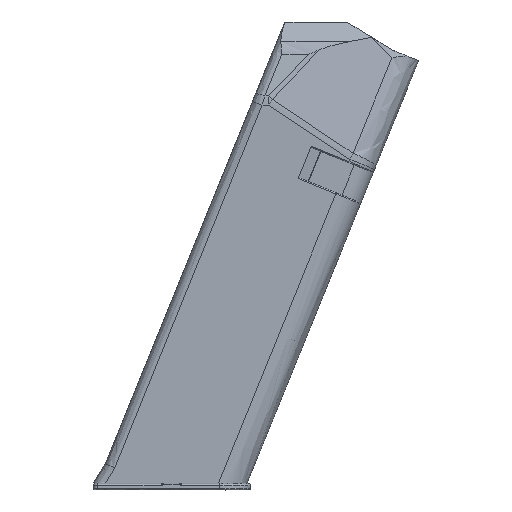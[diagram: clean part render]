
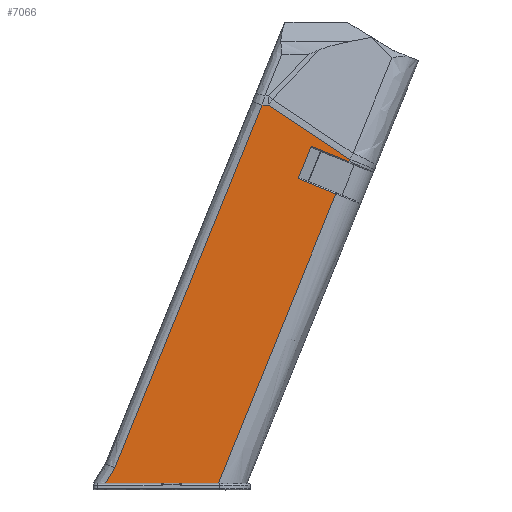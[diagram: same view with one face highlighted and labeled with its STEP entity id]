
A CAD part, top view. The second image highlights one B-rep face of the part: STEP entity #7066.
In plain terms, the highlighted planar face has unit normal (0, 0, 1).
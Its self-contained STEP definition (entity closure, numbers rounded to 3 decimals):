
#513=PLANE('',#7596);
#557=LINE('',#9516,#1223);
#1143=LINE('',#13379,#1809);
#1144=LINE('',#13438,#1810);
#1145=LINE('',#13441,#1811);
#1146=LINE('',#13443,#1812);
#1147=LINE('',#13445,#1813);
#1148=LINE('',#13447,#1814);
#1149=LINE('',#13449,#1815);
#1150=LINE('',#13451,#1816);
#1151=LINE('',#13452,#1817);
#1223=VECTOR('',#7720,982.236);
#1809=VECTOR('',#9110,10.);
#1810=VECTOR('',#9111,10.);
#1811=VECTOR('',#9114,1030.);
#1812=VECTOR('',#9115,975.);
#1813=VECTOR('',#9116,1030.);
#1814=VECTOR('',#9117,977.064);
#1815=VECTOR('',#9118,982.236);
#1816=VECTOR('',#9119,1030.);
#1817=VECTOR('',#9120,1028.422);
#2219=FACE_OUTER_BOUND('',#2621,.T.);
#2621=EDGE_LOOP('',(#6284,#6285,#6286,#6287,#6288,#6289,#6290,#6291,#6292,
#6293));
#2916=VERTEX_POINT('',#9513);
#2917=VERTEX_POINT('',#9515);
#3502=VERTEX_POINT('',#13372);
#3505=VERTEX_POINT('',#13377);
#3507=VERTEX_POINT('',#13440);
#3508=VERTEX_POINT('',#13442);
#3509=VERTEX_POINT('',#13444);
#3510=VERTEX_POINT('',#13446);
#3511=VERTEX_POINT('',#13448);
#3512=VERTEX_POINT('',#13450);
#3581=EDGE_CURVE('',#2916,#2917,#557,.T.);
#4474=EDGE_CURVE('',#3505,#3502,#1143,.T.);
#4478=EDGE_CURVE('',#2916,#3502,#1144,.T.);
#4479=EDGE_CURVE('',#3507,#3505,#1145,.T.);
#4480=EDGE_CURVE('',#3507,#3508,#1146,.T.);
#4481=EDGE_CURVE('',#3508,#3509,#1147,.T.);
#4482=EDGE_CURVE('',#3509,#3510,#1148,.T.);
#4483=EDGE_CURVE('',#3510,#3511,#1149,.T.);
#4484=EDGE_CURVE('',#3511,#3512,#1150,.T.);
#4485=EDGE_CURVE('',#3512,#2917,#1151,.T.);
#6284=ORIENTED_EDGE('',*,*,#3581,.F.);
#6285=ORIENTED_EDGE('',*,*,#4478,.T.);
#6286=ORIENTED_EDGE('',*,*,#4474,.F.);
#6287=ORIENTED_EDGE('',*,*,#4479,.F.);
#6288=ORIENTED_EDGE('',*,*,#4480,.T.);
#6289=ORIENTED_EDGE('',*,*,#4481,.T.);
#6290=ORIENTED_EDGE('',*,*,#4482,.T.);
#6291=ORIENTED_EDGE('',*,*,#4483,.T.);
#6292=ORIENTED_EDGE('',*,*,#4484,.T.);
#6293=ORIENTED_EDGE('',*,*,#4485,.T.);
#7066=ADVANCED_FACE('',(#2219),#513,.T.);
#7596=AXIS2_PLACEMENT_3D('',#13439,#9112,#9113);
#7720=DIRECTION('',(-1.,0.,0.));
#9110=DIRECTION('',(0.927,-0.376,0.));
#9111=DIRECTION('',(0.376,0.927,0.));
#9112=DIRECTION('center_axis',(0.,0.,1.));
#9113=DIRECTION('ref_axis',(0.927,-0.376,0.));
#9114=DIRECTION('',(-0.376,-0.927,0.));
#9115=DIRECTION('',(0.927,-0.376,0.));
#9116=DIRECTION('',(0.376,0.927,0.));
#9117=DIRECTION('',(-0.832,0.555,0.));
#9118=DIRECTION('',(-1.,0.,0.));
#9119=DIRECTION('',(-0.376,-0.927,0.));
#9120=DIRECTION('',(-0.522,-0.853,0.));
#9513=CARTESIAN_POINT('',(45.269,-1.412,11.526));
#9515=CARTESIAN_POINT('',(18.215,-1.4,11.526));
#9516=CARTESIAN_POINT('',(17.914,-1.399,11.526));
#13372=CARTESIAN_POINT('',(73.38,67.816,11.526));
#13377=CARTESIAN_POINT('',(64.346,71.484,11.526));
#13379=CARTESIAN_POINT('',(74.323,67.433,11.526));
#13438=CARTESIAN_POINT('',(73.322,67.675,11.526));
#13439=CARTESIAN_POINT('Origin',(76.21,66.363,11.526));
#13440=CARTESIAN_POINT('',(67.486,79.216,11.526));
#13441=CARTESIAN_POINT('',(67.389,78.977,11.526));
#13442=CARTESIAN_POINT('',(76.519,75.548,11.526));
#13443=CARTESIAN_POINT('',(53.032,85.085,11.526));
#13444=CARTESIAN_POINT('',(76.732,76.071,11.526));
#13445=CARTESIAN_POINT('',(76.242,74.863,11.526));
#13446=CARTESIAN_POINT('',(57.267,89.064,11.526));
#13447=CARTESIAN_POINT('',(80.763,73.381,11.526));
#13448=CARTESIAN_POINT('',(55.7,89.065,11.526));
#13449=CARTESIAN_POINT('',(21.28,89.081,11.526));
#13450=CARTESIAN_POINT('',(20.448,2.25,11.526));
#13451=CARTESIAN_POINT('',(20.532,2.456,11.526));
#13452=CARTESIAN_POINT('',(20.139,1.744,11.526));
